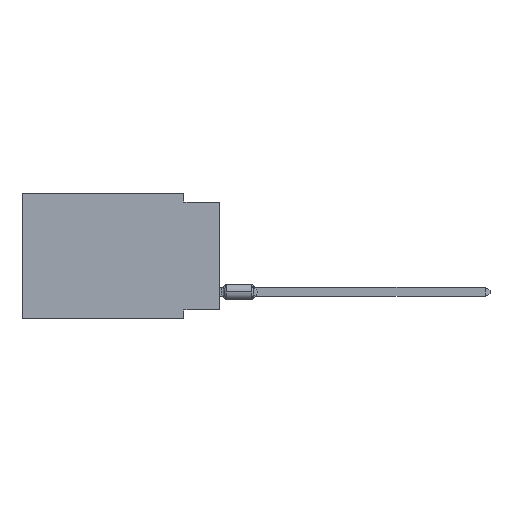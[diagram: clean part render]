
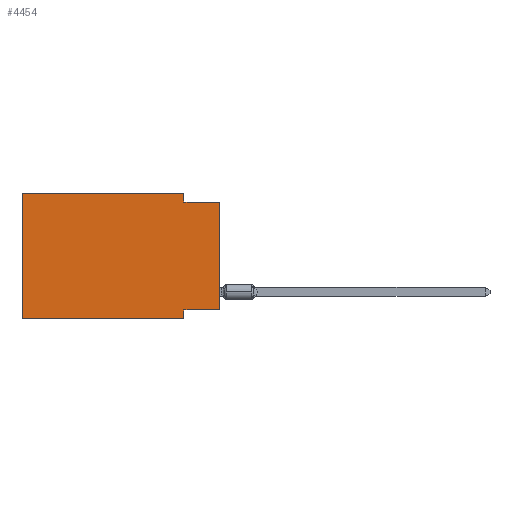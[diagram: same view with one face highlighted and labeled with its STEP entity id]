
A CAD part, left-side view. The second image highlights one B-rep face of the part: STEP entity #4454.
In plain terms, the highlighted planar face has unit normal (-1, 0, 0).
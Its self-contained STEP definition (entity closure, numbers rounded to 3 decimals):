
#234 = VECTOR ( 'NONE', #2011, 1000. ) ;
#295 = LINE ( 'NONE', #5509, #8636 ) ;
#383 = VERTEX_POINT ( 'NONE', #18368 ) ;
#404 = DIRECTION ( 'NONE',  ( 0., 0., 1. ) ) ;
#1526 = ORIENTED_EDGE ( 'NONE', *, *, #19930, .T. ) ;
#2011 = DIRECTION ( 'NONE',  ( 0., -1., 0. ) ) ;
#2142 = ORIENTED_EDGE ( 'NONE', *, *, #16071, .F. ) ;
#2228 = EDGE_CURVE ( 'NONE', #8614, #383, #8395, .T. ) ;
#2894 = VERTEX_POINT ( 'NONE', #16386 ) ;
#2916 = ORIENTED_EDGE ( 'NONE', *, *, #10737, .F. ) ;
#3285 = VERTEX_POINT ( 'NONE', #17939 ) ;
#3652 = EDGE_CURVE ( 'NONE', #16525, #17438, #19507, .T. ) ;
#3945 = CARTESIAN_POINT ( 'NONE',  ( 0., 0., -0.635 ) ) ;
#4244 = DIRECTION ( 'NONE',  ( 0., 0., -1. ) ) ;
#4454 = ADVANCED_FACE ( 'NONE', ( #11273 ), #21674, .F. ) ;
#4612 = DIRECTION ( 'NONE',  ( 0., -1., 0. ) ) ;
#5509 = CARTESIAN_POINT ( 'NONE',  ( 0., 0., 0. ) ) ;
#5721 = VECTOR ( 'NONE', #18449, 1000. ) ;
#5839 = DIRECTION ( 'NONE',  ( 0., 1., 0. ) ) ;
#6209 = ORIENTED_EDGE ( 'NONE', *, *, #2228, .F. ) ;
#6595 = EDGE_CURVE ( 'NONE', #8614, #17438, #11335, .T. ) ;
#6699 = ORIENTED_EDGE ( 'NONE', *, *, #18608, .F. ) ;
#6952 = ORIENTED_EDGE ( 'NONE', *, *, #20121, .F. ) ;
#7024 = ORIENTED_EDGE ( 'NONE', *, *, #6595, .T. ) ;
#7893 = CARTESIAN_POINT ( 'NONE',  ( 0., 2.54, 0. ) ) ;
#7894 = VECTOR ( 'NONE', #5839, 1000. ) ;
#8395 = LINE ( 'NONE', #13586, #8480 ) ;
#8480 = VECTOR ( 'NONE', #10196, 1000. ) ;
#8614 = VERTEX_POINT ( 'NONE', #19773 ) ;
#8634 = VERTEX_POINT ( 'NONE', #7893 ) ;
#8636 = VECTOR ( 'NONE', #404, 1000. ) ;
#9404 = EDGE_LOOP ( 'NONE', ( #1526, #6699, #2916, #2142, #6209, #7024, #19870, #6952 ) ) ;
#10196 = DIRECTION ( 'NONE',  ( 0., 0., 1. ) ) ;
#10737 = EDGE_CURVE ( 'NONE', #8634, #2894, #21434, .T. ) ;
#11027 = DIRECTION ( 'NONE',  ( 0., 0., -1. ) ) ;
#11135 = CARTESIAN_POINT ( 'NONE',  ( 0., 2.54, -8.89 ) ) ;
#11273 = FACE_OUTER_BOUND ( 'NONE', #9404, .T. ) ;
#11335 = LINE ( 'NONE', #11559, #5721 ) ;
#11559 = CARTESIAN_POINT ( 'NONE',  ( 0., 13.97, -8.89 ) ) ;
#12088 = CARTESIAN_POINT ( 'NONE',  ( 0., 13.97, 0. ) ) ;
#12517 = AXIS2_PLACEMENT_3D ( 'NONE', #18279, #14787, #12858 ) ;
#12628 = CARTESIAN_POINT ( 'NONE',  ( 0., 0., -8.255 ) ) ;
#12858 = DIRECTION ( 'NONE',  ( 0., 0., -1. ) ) ;
#13586 = CARTESIAN_POINT ( 'NONE',  ( 0., 13.97, 0. ) ) ;
#14787 = DIRECTION ( 'NONE',  ( 1., 0., 0. ) ) ;
#16071 = EDGE_CURVE ( 'NONE', #383, #8634, #20902, .T. ) ;
#16126 = CARTESIAN_POINT ( 'NONE',  ( 0., 2.54, 0. ) ) ;
#16259 = CARTESIAN_POINT ( 'NONE',  ( 0., 2.54, -8.89 ) ) ;
#16363 = VECTOR ( 'NONE', #4244, 1000. ) ;
#16386 = CARTESIAN_POINT ( 'NONE',  ( 0., 2.54, -0.635 ) ) ;
#16525 = VERTEX_POINT ( 'NONE', #20988 ) ;
#16590 = CARTESIAN_POINT ( 'NONE',  ( 0., 0., -0.635 ) ) ;
#17035 = LINE ( 'NONE', #16590, #18691 ) ;
#17311 = VERTEX_POINT ( 'NONE', #3945 ) ;
#17438 = VERTEX_POINT ( 'NONE', #16259 ) ;
#17939 = CARTESIAN_POINT ( 'NONE',  ( 0., 0., -8.255 ) ) ;
#18279 = CARTESIAN_POINT ( 'NONE',  ( 0., 13.97, 0. ) ) ;
#18368 = CARTESIAN_POINT ( 'NONE',  ( 0., 13.97, 0. ) ) ;
#18449 = DIRECTION ( 'NONE',  ( 0., -1., 0. ) ) ;
#18608 = EDGE_CURVE ( 'NONE', #2894, #17311, #17035, .T. ) ;
#18691 = VECTOR ( 'NONE', #4612, 1000. ) ;
#19362 = VECTOR ( 'NONE', #11027, 1000. ) ;
#19507 = LINE ( 'NONE', #11135, #19362 ) ;
#19773 = CARTESIAN_POINT ( 'NONE',  ( 0., 13.97, -8.89 ) ) ;
#19870 = ORIENTED_EDGE ( 'NONE', *, *, #3652, .F. ) ;
#19930 = EDGE_CURVE ( 'NONE', #3285, #17311, #295, .T. ) ;
#20121 = EDGE_CURVE ( 'NONE', #3285, #16525, #21438, .T. ) ;
#20902 = LINE ( 'NONE', #12088, #234 ) ;
#20988 = CARTESIAN_POINT ( 'NONE',  ( 0., 2.54, -8.255 ) ) ;
#21434 = LINE ( 'NONE', #16126, #16363 ) ;
#21438 = LINE ( 'NONE', #12628, #7894 ) ;
#21674 = PLANE ( 'NONE',  #12517 ) ;
